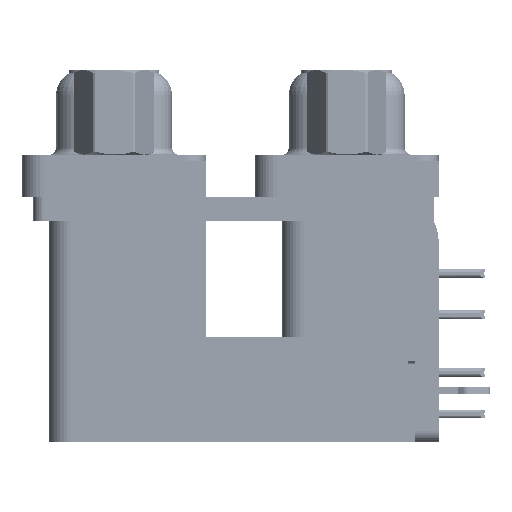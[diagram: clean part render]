
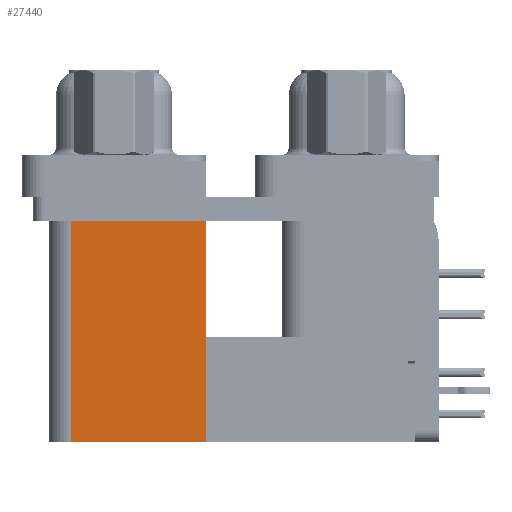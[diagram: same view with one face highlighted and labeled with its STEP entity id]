
A CAD part, left-side view. The second image highlights one B-rep face of the part: STEP entity #27440.
In plain terms, the highlighted planar face has unit normal (-1, 0, 0).
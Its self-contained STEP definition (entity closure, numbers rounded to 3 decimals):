
#3610 = EDGE_CURVE ( 'NONE', #69477, #72516, #28557, .T. ) ;
#4699 = CARTESIAN_POINT ( 'NONE',  ( 3.79, 18.8, -19.2 ) ) ;
#7836 = DIRECTION ( 'NONE',  ( 0., 1., 0. ) ) ;
#10444 = LINE ( 'NONE', #41618, #24655 ) ;
#15342 = EDGE_CURVE ( 'NONE', #26429, #70527, #10444, .T. ) ;
#15703 = PLANE ( 'NONE',  #21083 ) ;
#16664 = CARTESIAN_POINT ( 'NONE',  ( 3.79, 18.8, -19.2 ) ) ;
#20782 = CARTESIAN_POINT ( 'NONE',  ( 3.79, 9.6, -2.5 ) ) ;
#21083 = AXIS2_PLACEMENT_3D ( 'NONE', #65351, #59212, #33747 ) ;
#22575 = LINE ( 'NONE', #47576, #35656 ) ;
#24655 = VECTOR ( 'NONE', #48178, 1000. ) ;
#26429 = VERTEX_POINT ( 'NONE', #54235 ) ;
#27440 = ADVANCED_FACE ( 'NONE', ( #28010 ), #15703, .F. ) ;
#28010 = FACE_OUTER_BOUND ( 'NONE', #28627, .T. ) ;
#28557 = LINE ( 'NONE', #16664, #52522 ) ;
#28627 = EDGE_LOOP ( 'NONE', ( #31237, #58944, #56581, #46738 ) ) ;
#29401 = EDGE_CURVE ( 'NONE', #26429, #69477, #22575, .T. ) ;
#31237 = ORIENTED_EDGE ( 'NONE', *, *, #70052, .T. ) ;
#33747 = DIRECTION ( 'NONE',  ( 0., 0., -1. ) ) ;
#35656 = VECTOR ( 'NONE', #41415, 1000. ) ;
#40223 = LINE ( 'NONE', #64073, #62825 ) ;
#41415 = DIRECTION ( 'NONE',  ( 0., 1., 0. ) ) ;
#41618 = CARTESIAN_POINT ( 'NONE',  ( 3.79, 9.6, -19.2 ) ) ;
#46738 = ORIENTED_EDGE ( 'NONE', *, *, #15342, .T. ) ;
#47576 = CARTESIAN_POINT ( 'NONE',  ( 3.79, 9.6, -19.2 ) ) ;
#48178 = DIRECTION ( 'NONE',  ( 0., 0., 1. ) ) ;
#48784 = CARTESIAN_POINT ( 'NONE',  ( 3.79, 18.8, -2.5 ) ) ;
#52522 = VECTOR ( 'NONE', #53176, 1000. ) ;
#53176 = DIRECTION ( 'NONE',  ( 0., 0., 1. ) ) ;
#54235 = CARTESIAN_POINT ( 'NONE',  ( 3.79, 9.6, -19.2 ) ) ;
#56581 = ORIENTED_EDGE ( 'NONE', *, *, #29401, .F. ) ;
#58944 = ORIENTED_EDGE ( 'NONE', *, *, #3610, .F. ) ;
#59212 = DIRECTION ( 'NONE',  ( 1., 0., 0. ) ) ;
#62825 = VECTOR ( 'NONE', #7836, 1000. ) ;
#64073 = CARTESIAN_POINT ( 'NONE',  ( 3.79, 9.6, -2.5 ) ) ;
#65351 = CARTESIAN_POINT ( 'NONE',  ( 3.79, 9.6, -19.2 ) ) ;
#69477 = VERTEX_POINT ( 'NONE', #4699 ) ;
#70052 = EDGE_CURVE ( 'NONE', #70527, #72516, #40223, .T. ) ;
#70527 = VERTEX_POINT ( 'NONE', #20782 ) ;
#72516 = VERTEX_POINT ( 'NONE', #48784 ) ;
